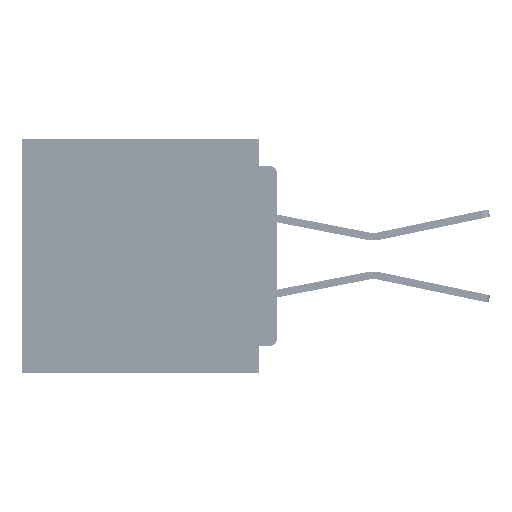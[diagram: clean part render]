
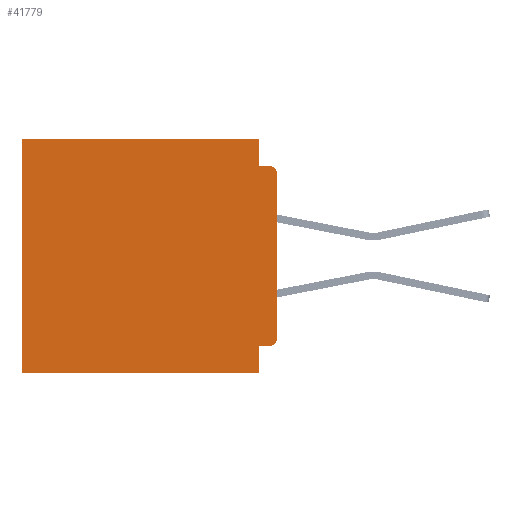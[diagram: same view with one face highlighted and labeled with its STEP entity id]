
A CAD part, left-side view. The second image highlights one B-rep face of the part: STEP entity #41779.
In plain terms, the highlighted planar face has unit normal (-1, 0, 0).
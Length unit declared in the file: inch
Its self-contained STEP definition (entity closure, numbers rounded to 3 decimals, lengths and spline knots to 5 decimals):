
#1294 = CARTESIAN_POINT ( 'NONE',  ( 0.3, 0.015, -0.06 ) ) ;
#2897 = EDGE_CURVE ( 'NONE', #35455, #68808, #69064, .T. ) ;
#4664 = CARTESIAN_POINT ( 'NONE',  ( 0.3, 0.031, 0. ) ) ;
#4695 = AXIS2_PLACEMENT_3D ( 'NONE', #1294, #39195, #6739 ) ;
#5163 = CIRCLE ( 'NONE', #4695, 0.015 ) ;
#5708 = VERTEX_POINT ( 'NONE', #21162 ) ;
#5877 = EDGE_CURVE ( 'NONE', #39797, #57917, #5163, .T. ) ;
#5892 = LINE ( 'NONE', #46068, #31280 ) ;
#6591 = VECTOR ( 'NONE', #22885, 39.37008 ) ;
#6739 = DIRECTION ( 'NONE',  ( 0., 0., -1. ) ) ;
#7063 = VERTEX_POINT ( 'NONE', #69242 ) ;
#8020 = AXIS2_PLACEMENT_3D ( 'NONE', #27994, #65863, #33459 ) ;
#9228 = VECTOR ( 'NONE', #34815, 39.37008 ) ;
#10118 = LINE ( 'NONE', #66300, #37237 ) ;
#10371 = CARTESIAN_POINT ( 'NONE',  ( 0.3, 0., -0.4 ) ) ;
#10843 = EDGE_CURVE ( 'NONE', #29460, #66114, #10118, .T. ) ;
#10974 = CARTESIAN_POINT ( 'NONE',  ( 0.3, 0.031, -0.4 ) ) ;
#13566 = ORIENTED_EDGE ( 'NONE', *, *, #38707, .F. ) ;
#13584 = DIRECTION ( 'NONE',  ( 0., -1., 0. ) ) ;
#15154 = ORIENTED_EDGE ( 'NONE', *, *, #10843, .F. ) ;
#16966 = ORIENTED_EDGE ( 'NONE', *, *, #2897, .F. ) ;
#19139 = EDGE_CURVE ( 'NONE', #69261, #68808, #21900, .T. ) ;
#19407 = CARTESIAN_POINT ( 'NONE',  ( 0.3, 0.015, -0.34 ) ) ;
#21162 = CARTESIAN_POINT ( 'NONE',  ( 0.3, 0.031, 0. ) ) ;
#21900 = LINE ( 'NONE', #56406, #9228 ) ;
#22885 = DIRECTION ( 'NONE',  ( 0., 0., -1. ) ) ;
#23306 = DIRECTION ( 'NONE',  ( 0., 1., 0. ) ) ;
#23503 = CARTESIAN_POINT ( 'NONE',  ( 0.3, 0.437, 0. ) ) ;
#24844 = DIRECTION ( 'NONE',  ( 0., 0., -1. ) ) ;
#25168 = CARTESIAN_POINT ( 'NONE',  ( 0.3, 0.015, -0.045 ) ) ;
#25594 = VECTOR ( 'NONE', #23306, 39.37008 ) ;
#26183 = CARTESIAN_POINT ( 'NONE',  ( 0.3, 0.031, -0.355 ) ) ;
#26557 = ORIENTED_EDGE ( 'NONE', *, *, #63397, .T. ) ;
#27286 = DIRECTION ( 'NONE',  ( 0., 0., -1. ) ) ;
#27994 = CARTESIAN_POINT ( 'NONE',  ( 0.3, 0., -0.4 ) ) ;
#28435 = DIRECTION ( 'NONE',  ( 0., 1., 0. ) ) ;
#29339 = LINE ( 'NONE', #10974, #58187 ) ;
#29460 = VERTEX_POINT ( 'NONE', #50471 ) ;
#31280 = VECTOR ( 'NONE', #13584, 39.37008 ) ;
#31971 = LINE ( 'NONE', #33785, #6591 ) ;
#33459 = DIRECTION ( 'NONE',  ( 0., 0., -1. ) ) ;
#33785 = CARTESIAN_POINT ( 'NONE',  ( 0.3, 0., -0.4 ) ) ;
#34210 = CARTESIAN_POINT ( 'NONE',  ( 0.3, 0., 0. ) ) ;
#34815 = DIRECTION ( 'NONE',  ( 0., 0., -1. ) ) ;
#35455 = VERTEX_POINT ( 'NONE', #52986 ) ;
#35708 = CIRCLE ( 'NONE', #35854, 0.015 ) ;
#35854 = AXIS2_PLACEMENT_3D ( 'NONE', #19407, #57335, #24844 ) ;
#37237 = VECTOR ( 'NONE', #28435, 39.37008 ) ;
#38707 = EDGE_CURVE ( 'NONE', #7063, #57917, #5892, .T. ) ;
#39195 = DIRECTION ( 'NONE',  ( -1., 0., 0. ) ) ;
#39797 = VERTEX_POINT ( 'NONE', #55185 ) ;
#39851 = EDGE_CURVE ( 'NONE', #39797, #66496, #31971, .T. ) ;
#40053 = LINE ( 'NONE', #34210, #25594 ) ;
#40414 = ORIENTED_EDGE ( 'NONE', *, *, #19139, .T. ) ;
#40769 = ORIENTED_EDGE ( 'NONE', *, *, #48852, .F. ) ;
#41779 = ADVANCED_FACE ( 'NONE', ( #64714 ), #60490, .F. ) ;
#41842 = ORIENTED_EDGE ( 'NONE', *, *, #39851, .F. ) ;
#42569 = DIRECTION ( 'NONE',  ( 0., 0., -1. ) ) ;
#46068 = CARTESIAN_POINT ( 'NONE',  ( 0.3, 0., -0.045 ) ) ;
#47687 = EDGE_CURVE ( 'NONE', #66114, #35455, #29339, .T. ) ;
#48852 = EDGE_CURVE ( 'NONE', #5708, #7063, #64744, .T. ) ;
#50431 = VECTOR ( 'NONE', #42569, 39.37008 ) ;
#50471 = CARTESIAN_POINT ( 'NONE',  ( 0.3, 0.015, -0.355 ) ) ;
#52329 = CARTESIAN_POINT ( 'NONE',  ( 0.3, 0.437, -0.4 ) ) ;
#52352 = EDGE_CURVE ( 'NONE', #29460, #66496, #35708, .T. ) ;
#52986 = CARTESIAN_POINT ( 'NONE',  ( 0.3, 0.031, -0.4 ) ) ;
#54795 = VECTOR ( 'NONE', #66538, 39.37008 ) ;
#55185 = CARTESIAN_POINT ( 'NONE',  ( 0.3, 0., -0.06 ) ) ;
#55454 = ORIENTED_EDGE ( 'NONE', *, *, #47687, .F. ) ;
#55549 = ORIENTED_EDGE ( 'NONE', *, *, #52352, .T. ) ;
#56406 = CARTESIAN_POINT ( 'NONE',  ( 0.3, 0.437, -0.4 ) ) ;
#57335 = DIRECTION ( 'NONE',  ( -1., 0., 0. ) ) ;
#57421 = EDGE_LOOP ( 'NONE', ( #41842, #62466, #13566, #40769, #26557, #40414, #16966, #55454, #15154, #55549 ) ) ;
#57917 = VERTEX_POINT ( 'NONE', #25168 ) ;
#58187 = VECTOR ( 'NONE', #27286, 39.37008 ) ;
#60490 = PLANE ( 'NONE',  #8020 ) ;
#62466 = ORIENTED_EDGE ( 'NONE', *, *, #5877, .T. ) ;
#63397 = EDGE_CURVE ( 'NONE', #5708, #69261, #40053, .T. ) ;
#64714 = FACE_OUTER_BOUND ( 'NONE', #57421, .T. ) ;
#64744 = LINE ( 'NONE', #4664, #50431 ) ;
#65863 = DIRECTION ( 'NONE',  ( 1., 0., 0. ) ) ;
#66114 = VERTEX_POINT ( 'NONE', #26183 ) ;
#66300 = CARTESIAN_POINT ( 'NONE',  ( 0.3, 0., -0.355 ) ) ;
#66496 = VERTEX_POINT ( 'NONE', #67750 ) ;
#66538 = DIRECTION ( 'NONE',  ( 0., 1., 0. ) ) ;
#67750 = CARTESIAN_POINT ( 'NONE',  ( 0.3, 0., -0.34 ) ) ;
#68808 = VERTEX_POINT ( 'NONE', #52329 ) ;
#69064 = LINE ( 'NONE', #10371, #54795 ) ;
#69242 = CARTESIAN_POINT ( 'NONE',  ( 0.3, 0.031, -0.045 ) ) ;
#69261 = VERTEX_POINT ( 'NONE', #23503 ) ;
